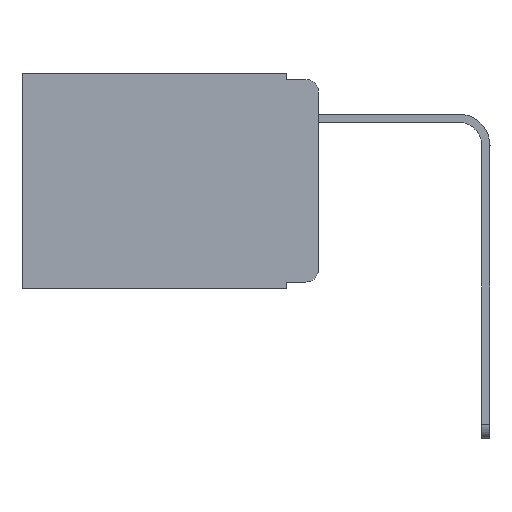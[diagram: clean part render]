
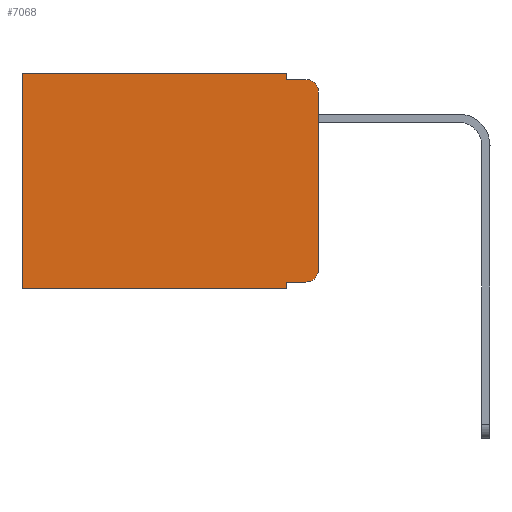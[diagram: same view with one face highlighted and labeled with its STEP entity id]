
A CAD part, left-side view. The second image highlights one B-rep face of the part: STEP entity #7068.
In plain terms, the highlighted planar face has unit normal (-1, 0, 0).
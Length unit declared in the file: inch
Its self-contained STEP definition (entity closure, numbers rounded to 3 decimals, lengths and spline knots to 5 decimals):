
#107 = VERTEX_POINT ( 'NONE', #3070 ) ;
#272 = CARTESIAN_POINT ( 'NONE',  ( 0.298, 0.473, 0. ) ) ;
#391 = DIRECTION ( 'NONE',  ( 0., 0., -1. ) ) ;
#424 = CARTESIAN_POINT ( 'NONE',  ( 0.298, 0., 0. ) ) ;
#628 = DIRECTION ( 'NONE',  ( -1., 0., 0. ) ) ;
#644 = EDGE_CURVE ( 'NONE', #5473, #7133, #8802, .T. ) ;
#692 = CARTESIAN_POINT ( 'NONE',  ( 0.298, 0.02, -0.01 ) ) ;
#1008 = VERTEX_POINT ( 'NONE', #8666 ) ;
#1078 = VECTOR ( 'NONE', #6157, 39.37008 ) ;
#1100 = CARTESIAN_POINT ( 'NONE',  ( 0.298, 0.051, -0.333 ) ) ;
#1134 = ORIENTED_EDGE ( 'NONE', *, *, #7024, .F. ) ;
#1245 = VECTOR ( 'NONE', #1354, 39.37008 ) ;
#1262 = LINE ( 'NONE', #3966, #1078 ) ;
#1288 = AXIS2_PLACEMENT_3D ( 'NONE', #6988, #4240, #7050 ) ;
#1348 = DIRECTION ( 'NONE',  ( 0., 0., -1. ) ) ;
#1354 = DIRECTION ( 'NONE',  ( 0., 0., -1. ) ) ;
#1526 = ORIENTED_EDGE ( 'NONE', *, *, #9256, .F. ) ;
#1527 = VECTOR ( 'NONE', #5405, 39.37008 ) ;
#1610 = VERTEX_POINT ( 'NONE', #8686 ) ;
#1824 = DIRECTION ( 'NONE',  ( 0., 0., -1. ) ) ;
#1880 = EDGE_CURVE ( 'NONE', #5775, #7133, #4162, .T. ) ;
#2091 = VERTEX_POINT ( 'NONE', #692 ) ;
#2123 = LINE ( 'NONE', #424, #5752 ) ;
#2166 = CARTESIAN_POINT ( 'NONE',  ( 0.298, 0.473, 0. ) ) ;
#2537 = CARTESIAN_POINT ( 'NONE',  ( 0.298, 0.051, -0.01 ) ) ;
#2788 = LINE ( 'NONE', #4139, #3345 ) ;
#3070 = CARTESIAN_POINT ( 'NONE',  ( 0.298, 0.051, -0.01 ) ) ;
#3072 = VERTEX_POINT ( 'NONE', #6169 ) ;
#3194 = EDGE_CURVE ( 'NONE', #8123, #1008, #2788, .T. ) ;
#3310 = CARTESIAN_POINT ( 'NONE',  ( 0.298, 0.02, -0.03 ) ) ;
#3345 = VECTOR ( 'NONE', #9199, 39.37008 ) ;
#3847 = VECTOR ( 'NONE', #5534, 39.37008 ) ;
#3926 = DIRECTION ( 'NONE',  ( -1., 0., 0. ) ) ;
#3966 = CARTESIAN_POINT ( 'NONE',  ( 0.298, 0., 0. ) ) ;
#3975 = LINE ( 'NONE', #4321, #1245 ) ;
#4048 = CARTESIAN_POINT ( 'NONE',  ( 0.298, 0.051, -0.343 ) ) ;
#4139 = CARTESIAN_POINT ( 'NONE',  ( 0.298, 0.051, -0.333 ) ) ;
#4162 = LINE ( 'NONE', #272, #6431 ) ;
#4240 = DIRECTION ( 'NONE',  ( 1., 0., 0. ) ) ;
#4321 = CARTESIAN_POINT ( 'NONE',  ( 0.298, 0.051, 0. ) ) ;
#4355 = LINE ( 'NONE', #2537, #7298 ) ;
#4418 = AXIS2_PLACEMENT_3D ( 'NONE', #3310, #3926, #1824 ) ;
#4927 = ORIENTED_EDGE ( 'NONE', *, *, #5027, .F. ) ;
#4971 = FACE_OUTER_BOUND ( 'NONE', #5875, .T. ) ;
#4985 = CARTESIAN_POINT ( 'NONE',  ( 0.298, 0.02, -0.313 ) ) ;
#5027 = EDGE_CURVE ( 'NONE', #8123, #5473, #3975, .T. ) ;
#5243 = AXIS2_PLACEMENT_3D ( 'NONE', #4985, #628, #1348 ) ;
#5254 = CIRCLE ( 'NONE', #4418, 0.02 ) ;
#5324 = ORIENTED_EDGE ( 'NONE', *, *, #5432, .F. ) ;
#5405 = DIRECTION ( 'NONE',  ( 0., 1., 0. ) ) ;
#5432 = EDGE_CURVE ( 'NONE', #6839, #107, #7146, .T. ) ;
#5473 = VERTEX_POINT ( 'NONE', #4048 ) ;
#5534 = DIRECTION ( 'NONE',  ( 0., 0., -1. ) ) ;
#5560 = CARTESIAN_POINT ( 'NONE',  ( 0.298, 0.473, -0.343 ) ) ;
#5700 = ORIENTED_EDGE ( 'NONE', *, *, #1880, .T. ) ;
#5752 = VECTOR ( 'NONE', #391, 39.37008 ) ;
#5775 = VERTEX_POINT ( 'NONE', #2166 ) ;
#5800 = ORIENTED_EDGE ( 'NONE', *, *, #7977, .T. ) ;
#5875 = EDGE_LOOP ( 'NONE', ( #1134, #9053, #1526, #5324, #5800, #5700, #7567, #4927, #6630, #5988 ) ) ;
#5988 = ORIENTED_EDGE ( 'NONE', *, *, #6598, .T. ) ;
#6157 = DIRECTION ( 'NONE',  ( 0., 1., 0. ) ) ;
#6169 = CARTESIAN_POINT ( 'NONE',  ( 0.298, 0., -0.03 ) ) ;
#6431 = VECTOR ( 'NONE', #6815, 39.37008 ) ;
#6598 = EDGE_CURVE ( 'NONE', #1008, #1610, #8240, .T. ) ;
#6630 = ORIENTED_EDGE ( 'NONE', *, *, #3194, .T. ) ;
#6815 = DIRECTION ( 'NONE',  ( 0., 0., -1. ) ) ;
#6839 = VERTEX_POINT ( 'NONE', #7526 ) ;
#6843 = DIRECTION ( 'NONE',  ( 0., -1., 0. ) ) ;
#6988 = CARTESIAN_POINT ( 'NONE',  ( 0.298, 0., 0. ) ) ;
#7024 = EDGE_CURVE ( 'NONE', #3072, #1610, #2123, .T. ) ;
#7050 = DIRECTION ( 'NONE',  ( 0., 0., -1. ) ) ;
#7068 = ADVANCED_FACE ( 'NONE', ( #4971 ), #9241, .F. ) ;
#7133 = VERTEX_POINT ( 'NONE', #5560 ) ;
#7146 = LINE ( 'NONE', #7685, #3847 ) ;
#7298 = VECTOR ( 'NONE', #6843, 39.37008 ) ;
#7526 = CARTESIAN_POINT ( 'NONE',  ( 0.298, 0.051, 0. ) ) ;
#7567 = ORIENTED_EDGE ( 'NONE', *, *, #644, .F. ) ;
#7652 = CARTESIAN_POINT ( 'NONE',  ( 0.298, 0., -0.343 ) ) ;
#7685 = CARTESIAN_POINT ( 'NONE',  ( 0.298, 0.051, 0. ) ) ;
#7977 = EDGE_CURVE ( 'NONE', #6839, #5775, #1262, .T. ) ;
#8123 = VERTEX_POINT ( 'NONE', #1100 ) ;
#8240 = CIRCLE ( 'NONE', #5243, 0.02 ) ;
#8666 = CARTESIAN_POINT ( 'NONE',  ( 0.298, 0.02, -0.333 ) ) ;
#8686 = CARTESIAN_POINT ( 'NONE',  ( 0.298, 0., -0.313 ) ) ;
#8802 = LINE ( 'NONE', #7652, #1527 ) ;
#9053 = ORIENTED_EDGE ( 'NONE', *, *, #9174, .T. ) ;
#9174 = EDGE_CURVE ( 'NONE', #3072, #2091, #5254, .T. ) ;
#9199 = DIRECTION ( 'NONE',  ( 0., -1., 0. ) ) ;
#9241 = PLANE ( 'NONE',  #1288 ) ;
#9256 = EDGE_CURVE ( 'NONE', #107, #2091, #4355, .T. ) ;
